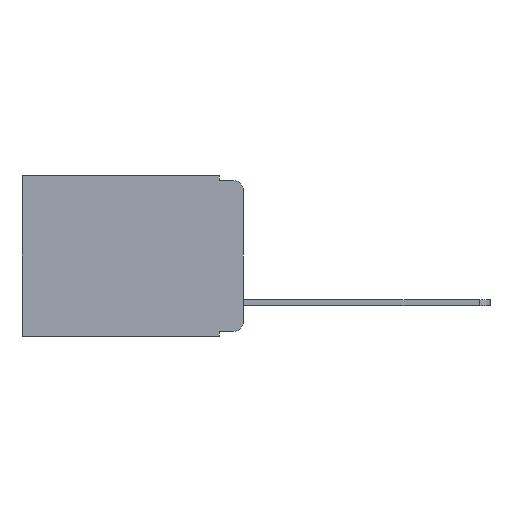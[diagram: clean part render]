
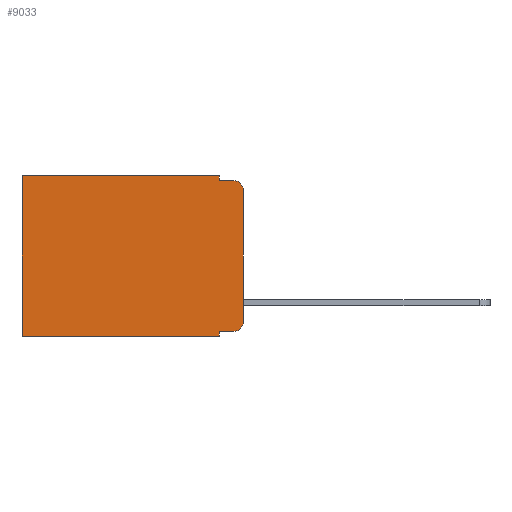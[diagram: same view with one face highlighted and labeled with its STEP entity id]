
A CAD part, left-side view. The second image highlights one B-rep face of the part: STEP entity #9033.
In plain terms, the highlighted planar face has unit normal (-1, 0, 0).
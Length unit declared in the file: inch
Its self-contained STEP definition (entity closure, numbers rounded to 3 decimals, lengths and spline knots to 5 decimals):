
#452 = CARTESIAN_POINT ( 'NONE',  ( 0.298, 0.051, -0.333 ) ) ;
#483 = VERTEX_POINT ( 'NONE', #4749 ) ;
#484 = CARTESIAN_POINT ( 'NONE',  ( 0.298, 0., 0. ) ) ;
#820 = ORIENTED_EDGE ( 'NONE', *, *, #6662, .F. ) ;
#836 = VERTEX_POINT ( 'NONE', #10844 ) ;
#963 = EDGE_CURVE ( 'NONE', #6726, #5281, #14637, .T. ) ;
#1298 = CIRCLE ( 'NONE', #5201, 0.02 ) ;
#1353 = LINE ( 'NONE', #1972, #12940 ) ;
#1877 = DIRECTION ( 'NONE',  ( -1., 0., 0. ) ) ;
#1945 = ORIENTED_EDGE ( 'NONE', *, *, #7874, .F. ) ;
#1972 = CARTESIAN_POINT ( 'NONE',  ( 0.298, 0.051, 0. ) ) ;
#2089 = DIRECTION ( 'NONE',  ( 0., -1., 0. ) ) ;
#2409 = LINE ( 'NONE', #16485, #6387 ) ;
#2692 = VECTOR ( 'NONE', #17743, 39.37008 ) ;
#3210 = DIRECTION ( 'NONE',  ( 0., 0., -1. ) ) ;
#3486 = CARTESIAN_POINT ( 'NONE',  ( 0.298, 0., -0.343 ) ) ;
#3965 = VECTOR ( 'NONE', #10679, 39.37008 ) ;
#4581 = DIRECTION ( 'NONE',  ( -1., 0., 0. ) ) ;
#4749 = CARTESIAN_POINT ( 'NONE',  ( 0.298, 0.051, 0. ) ) ;
#4788 = ORIENTED_EDGE ( 'NONE', *, *, #16768, .T. ) ;
#5096 = AXIS2_PLACEMENT_3D ( 'NONE', #5524, #18232, #9858 ) ;
#5107 = VERTEX_POINT ( 'NONE', #6944 ) ;
#5201 = AXIS2_PLACEMENT_3D ( 'NONE', #10618, #1877, #12044 ) ;
#5242 = ORIENTED_EDGE ( 'NONE', *, *, #11101, .T. ) ;
#5281 = VERTEX_POINT ( 'NONE', #6166 ) ;
#5429 = CARTESIAN_POINT ( 'NONE',  ( 0.298, 0., 0. ) ) ;
#5524 = CARTESIAN_POINT ( 'NONE',  ( 0.298, 0., 0. ) ) ;
#5782 = VERTEX_POINT ( 'NONE', #10184 ) ;
#5922 = ORIENTED_EDGE ( 'NONE', *, *, #963, .T. ) ;
#6166 = CARTESIAN_POINT ( 'NONE',  ( 0.298, 0.02, -0.01 ) ) ;
#6387 = VECTOR ( 'NONE', #6556, 39.37008 ) ;
#6388 = ORIENTED_EDGE ( 'NONE', *, *, #18559, .F. ) ;
#6556 = DIRECTION ( 'NONE',  ( 0., 0., -1. ) ) ;
#6609 = CARTESIAN_POINT ( 'NONE',  ( 0.298, 0.051, -0.01 ) ) ;
#6637 = FACE_OUTER_BOUND ( 'NONE', #8916, .T. ) ;
#6662 = EDGE_CURVE ( 'NONE', #12565, #5782, #9880, .T. ) ;
#6726 = VERTEX_POINT ( 'NONE', #8049 ) ;
#6745 = CARTESIAN_POINT ( 'NONE',  ( 0.298, 0.051, 0. ) ) ;
#6815 = VERTEX_POINT ( 'NONE', #11470 ) ;
#6944 = CARTESIAN_POINT ( 'NONE',  ( 0.298, 0.02, -0.333 ) ) ;
#7713 = EDGE_CURVE ( 'NONE', #483, #17914, #14275, .T. ) ;
#7874 = EDGE_CURVE ( 'NONE', #6726, #836, #9586, .T. ) ;
#8049 = CARTESIAN_POINT ( 'NONE',  ( 0.298, 0., -0.03 ) ) ;
#8244 = EDGE_CURVE ( 'NONE', #5107, #836, #1298, .T. ) ;
#8276 = DIRECTION ( 'NONE',  ( 0., 0., -1. ) ) ;
#8916 = EDGE_LOOP ( 'NONE', ( #1945, #5922, #6388, #17662, #18481, #4788, #820, #9964, #5242, #10860 ) ) ;
#9033 = ADVANCED_FACE ( 'NONE', ( #6637 ), #11218, .F. ) ;
#9586 = LINE ( 'NONE', #5429, #11554 ) ;
#9752 = VECTOR ( 'NONE', #17970, 39.37008 ) ;
#9858 = DIRECTION ( 'NONE',  ( 0., 0., -1. ) ) ;
#9880 = LINE ( 'NONE', #3486, #13222 ) ;
#9964 = ORIENTED_EDGE ( 'NONE', *, *, #12992, .F. ) ;
#10167 = LINE ( 'NONE', #6745, #9752 ) ;
#10184 = CARTESIAN_POINT ( 'NONE',  ( 0.298, 0.473, -0.343 ) ) ;
#10357 = AXIS2_PLACEMENT_3D ( 'NONE', #14566, #4581, #3210 ) ;
#10618 = CARTESIAN_POINT ( 'NONE',  ( 0.298, 0.02, -0.313 ) ) ;
#10679 = DIRECTION ( 'NONE',  ( 0., -1., 0. ) ) ;
#10844 = CARTESIAN_POINT ( 'NONE',  ( 0.298, 0., -0.313 ) ) ;
#10860 = ORIENTED_EDGE ( 'NONE', *, *, #8244, .T. ) ;
#11101 = EDGE_CURVE ( 'NONE', #13328, #5107, #11632, .T. ) ;
#11218 = PLANE ( 'NONE',  #5096 ) ;
#11470 = CARTESIAN_POINT ( 'NONE',  ( 0.298, 0.051, -0.01 ) ) ;
#11554 = VECTOR ( 'NONE', #8276, 39.37008 ) ;
#11632 = LINE ( 'NONE', #452, #3965 ) ;
#12044 = DIRECTION ( 'NONE',  ( 0., 0., -1. ) ) ;
#12565 = VERTEX_POINT ( 'NONE', #12755 ) ;
#12755 = CARTESIAN_POINT ( 'NONE',  ( 0.298, 0.051, -0.343 ) ) ;
#12940 = VECTOR ( 'NONE', #17747, 39.37008 ) ;
#12992 = EDGE_CURVE ( 'NONE', #13328, #12565, #1353, .T. ) ;
#13222 = VECTOR ( 'NONE', #15053, 39.37008 ) ;
#13328 = VERTEX_POINT ( 'NONE', #14342 ) ;
#14275 = LINE ( 'NONE', #484, #2692 ) ;
#14342 = CARTESIAN_POINT ( 'NONE',  ( 0.298, 0.051, -0.333 ) ) ;
#14566 = CARTESIAN_POINT ( 'NONE',  ( 0.298, 0.02, -0.03 ) ) ;
#14637 = CIRCLE ( 'NONE', #10357, 0.02 ) ;
#14943 = EDGE_CURVE ( 'NONE', #483, #6815, #10167, .T. ) ;
#15027 = LINE ( 'NONE', #6609, #18195 ) ;
#15053 = DIRECTION ( 'NONE',  ( 0., 1., 0. ) ) ;
#16324 = CARTESIAN_POINT ( 'NONE',  ( 0.298, 0.473, 0. ) ) ;
#16485 = CARTESIAN_POINT ( 'NONE',  ( 0.298, 0.473, 0. ) ) ;
#16768 = EDGE_CURVE ( 'NONE', #17914, #5782, #2409, .T. ) ;
#17662 = ORIENTED_EDGE ( 'NONE', *, *, #14943, .F. ) ;
#17743 = DIRECTION ( 'NONE',  ( 0., 1., 0. ) ) ;
#17747 = DIRECTION ( 'NONE',  ( 0., 0., -1. ) ) ;
#17914 = VERTEX_POINT ( 'NONE', #16324 ) ;
#17970 = DIRECTION ( 'NONE',  ( 0., 0., -1. ) ) ;
#18195 = VECTOR ( 'NONE', #2089, 39.37008 ) ;
#18232 = DIRECTION ( 'NONE',  ( 1., 0., 0. ) ) ;
#18481 = ORIENTED_EDGE ( 'NONE', *, *, #7713, .T. ) ;
#18559 = EDGE_CURVE ( 'NONE', #6815, #5281, #15027, .T. ) ;
